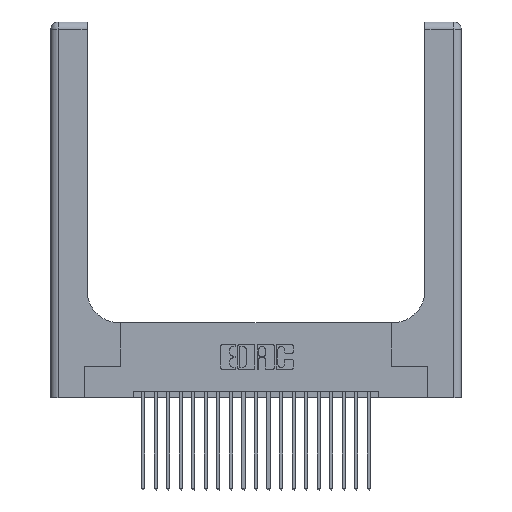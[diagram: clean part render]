
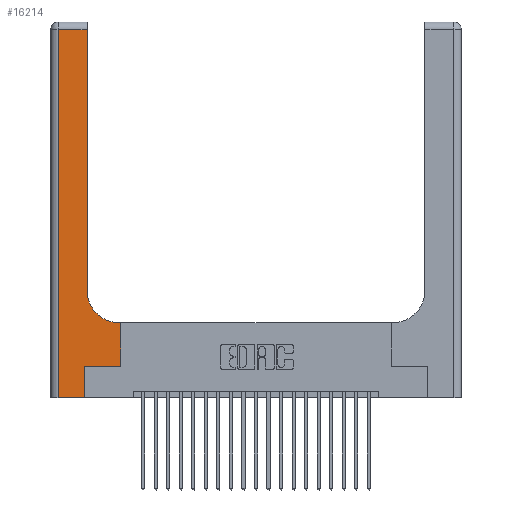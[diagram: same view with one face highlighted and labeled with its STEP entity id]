
A CAD part, top view. The second image highlights one B-rep face of the part: STEP entity #16214.
In plain terms, the highlighted planar face has unit normal (0, 0, 1).
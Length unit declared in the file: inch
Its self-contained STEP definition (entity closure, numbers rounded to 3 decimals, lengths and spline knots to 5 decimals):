
#60 = CARTESIAN_POINT ( 'NONE',  ( 0.06, 3., 0.37 ) ) ;
#177 = PLANE ( 'NONE',  #12384 ) ;
#616 = CARTESIAN_POINT ( 'NONE',  ( 0.06, 0., 0.37 ) ) ;
#865 = VERTEX_POINT ( 'NONE', #616 ) ;
#990 = ORIENTED_EDGE ( 'NONE', *, *, #4269, .T. ) ;
#1047 = CARTESIAN_POINT ( 'NONE',  ( 0.269, 0., 0.37 ) ) ;
#1429 = CARTESIAN_POINT ( 'NONE',  ( 0.2915, 3., 0.37 ) ) ;
#1451 = ORIENTED_EDGE ( 'NONE', *, *, #16896, .T. ) ;
#1745 = CARTESIAN_POINT ( 'NONE',  ( 0.2915, 0.85, 0.37 ) ) ;
#1925 = VECTOR ( 'NONE', #22857, 39.37008 ) ;
#2052 = VERTEX_POINT ( 'NONE', #14178 ) ;
#2071 = ORIENTED_EDGE ( 'NONE', *, *, #2509, .T. ) ;
#2215 = CARTESIAN_POINT ( 'NONE',  ( 0.5585, 0.25, 0.37 ) ) ;
#2370 = VERTEX_POINT ( 'NONE', #5182 ) ;
#2451 = VERTEX_POINT ( 'NONE', #1745 ) ;
#2509 = EDGE_CURVE ( 'NONE', #5598, #2370, #15734, .T. ) ;
#2878 = EDGE_CURVE ( 'NONE', #2451, #14689, #3726, .T. ) ;
#3153 = ORIENTED_EDGE ( 'NONE', *, *, #9417, .T. ) ;
#3288 = DIRECTION ( 'NONE',  ( 0., 1., 0. ) ) ;
#3323 = DIRECTION ( 'NONE',  ( -1., 0., 0. ) ) ;
#3594 = EDGE_CURVE ( 'NONE', #17616, #865, #19000, .T. ) ;
#3726 = LINE ( 'NONE', #1429, #22046 ) ;
#3929 = CARTESIAN_POINT ( 'NONE',  ( 0.5585, 0.25, 0.37 ) ) ;
#4226 = CARTESIAN_POINT ( 'NONE',  ( 0.5415, 0.85, 0.37 ) ) ;
#4269 = EDGE_CURVE ( 'NONE', #865, #7362, #19240, .T. ) ;
#4325 = VERTEX_POINT ( 'NONE', #10668 ) ;
#4436 = ORIENTED_EDGE ( 'NONE', *, *, #13629, .T. ) ;
#5123 = ORIENTED_EDGE ( 'NONE', *, *, #19688, .T. ) ;
#5182 = CARTESIAN_POINT ( 'NONE',  ( 0.5585, 0.6, 0.37 ) ) ;
#5266 = FACE_OUTER_BOUND ( 'NONE', #8527, .T. ) ;
#5598 = VERTEX_POINT ( 'NONE', #3929 ) ;
#6029 = DIRECTION ( 'NONE',  ( 1., 0., 0. ) ) ;
#7141 = AXIS2_PLACEMENT_3D ( 'NONE', #4226, #16670, #6029 ) ;
#7362 = VERTEX_POINT ( 'NONE', #1047 ) ;
#7948 = LINE ( 'NONE', #15814, #17418 ) ;
#8433 = ORIENTED_EDGE ( 'NONE', *, *, #2878, .T. ) ;
#8527 = EDGE_LOOP ( 'NONE', ( #8433, #3153, #11583, #990, #1451, #4436, #2071, #10674, #5123 ) ) ;
#9340 = DIRECTION ( 'NONE',  ( 0., 0., -1. ) ) ;
#9417 = EDGE_CURVE ( 'NONE', #14689, #17616, #9434, .T. ) ;
#9434 = LINE ( 'NONE', #12153, #13641 ) ;
#10206 = VECTOR ( 'NONE', #14633, 39.37008 ) ;
#10467 = CARTESIAN_POINT ( 'NONE',  ( 0.269, 0.25, 0.37 ) ) ;
#10668 = CARTESIAN_POINT ( 'NONE',  ( 0.5415, 0.6, 0.37 ) ) ;
#10674 = ORIENTED_EDGE ( 'NONE', *, *, #11141, .T. ) ;
#10924 = LINE ( 'NONE', #10467, #1925 ) ;
#11141 = EDGE_CURVE ( 'NONE', #2370, #4325, #7948, .T. ) ;
#11301 = CIRCLE ( 'NONE', #7141, 0.25 ) ;
#11583 = ORIENTED_EDGE ( 'NONE', *, *, #3594, .T. ) ;
#12054 = CARTESIAN_POINT ( 'NONE',  ( 0.2915, 2.94, 0.37 ) ) ;
#12153 = CARTESIAN_POINT ( 'NONE',  ( 0., 2.94, 0.37 ) ) ;
#12308 = CARTESIAN_POINT ( 'NONE',  ( 0., 0., 0.37 ) ) ;
#12384 = AXIS2_PLACEMENT_3D ( 'NONE', #19954, #9340, #21731 ) ;
#13629 = EDGE_CURVE ( 'NONE', #2052, #5598, #10924, .T. ) ;
#13641 = VECTOR ( 'NONE', #22738, 39.37008 ) ;
#13796 = VECTOR ( 'NONE', #18900, 39.37008 ) ;
#14129 = DIRECTION ( 'NONE',  ( 1., 0., 0. ) ) ;
#14178 = CARTESIAN_POINT ( 'NONE',  ( 0.269, 0.25, 0.37 ) ) ;
#14633 = DIRECTION ( 'NONE',  ( 0., 1., 0. ) ) ;
#14689 = VERTEX_POINT ( 'NONE', #12054 ) ;
#14832 = DIRECTION ( 'NONE',  ( 0., 1., 0. ) ) ;
#15364 = CARTESIAN_POINT ( 'NONE',  ( 0.06, 2.94, 0.37 ) ) ;
#15734 = LINE ( 'NONE', #2215, #19853 ) ;
#15814 = CARTESIAN_POINT ( 'NONE',  ( 0.2915, 0.6, 0.37 ) ) ;
#16214 = ADVANCED_FACE ( 'NONE', ( #5266 ), #177, .F. ) ;
#16670 = DIRECTION ( 'NONE',  ( 0., 0., -1. ) ) ;
#16896 = EDGE_CURVE ( 'NONE', #7362, #2052, #20184, .T. ) ;
#17418 = VECTOR ( 'NONE', #3323, 39.37008 ) ;
#17616 = VERTEX_POINT ( 'NONE', #15364 ) ;
#18156 = CARTESIAN_POINT ( 'NONE',  ( 0.269, 0., 0.37 ) ) ;
#18900 = DIRECTION ( 'NONE',  ( 0., -1., 0. ) ) ;
#19000 = LINE ( 'NONE', #60, #13796 ) ;
#19240 = LINE ( 'NONE', #12308, #22861 ) ;
#19688 = EDGE_CURVE ( 'NONE', #4325, #2451, #11301, .T. ) ;
#19853 = VECTOR ( 'NONE', #14832, 39.37008 ) ;
#19954 = CARTESIAN_POINT ( 'NONE',  ( 0., 3., 0.37 ) ) ;
#20184 = LINE ( 'NONE', #18156, #10206 ) ;
#21731 = DIRECTION ( 'NONE',  ( -1., 0., 0. ) ) ;
#22046 = VECTOR ( 'NONE', #3288, 39.37008 ) ;
#22738 = DIRECTION ( 'NONE',  ( -1., 0., 0. ) ) ;
#22857 = DIRECTION ( 'NONE',  ( 1., 0., 0. ) ) ;
#22861 = VECTOR ( 'NONE', #14129, 39.37008 ) ;
